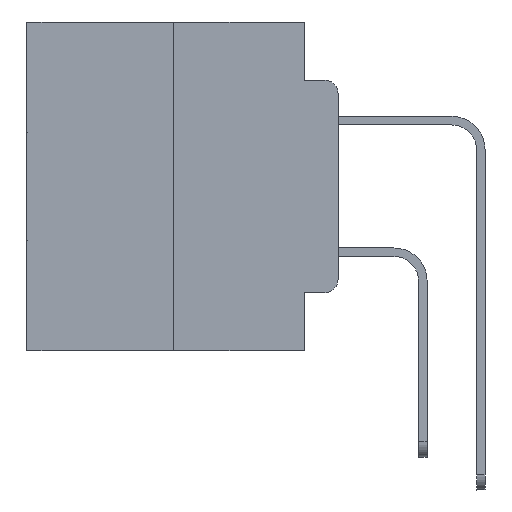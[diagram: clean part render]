
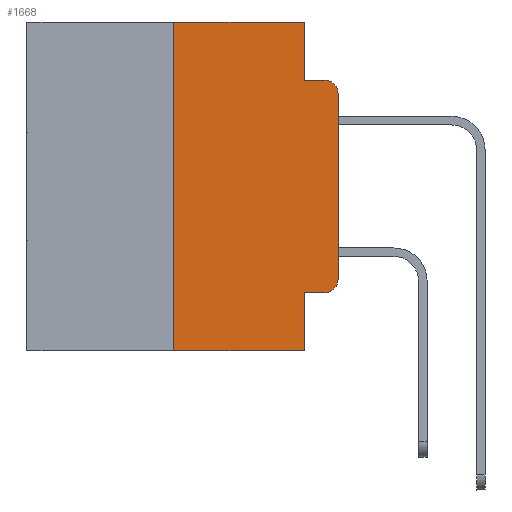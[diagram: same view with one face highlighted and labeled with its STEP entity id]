
A CAD part, left-side view. The second image highlights one B-rep face of the part: STEP entity #1668.
In plain terms, the highlighted planar face has unit normal (-1, 0, 0).
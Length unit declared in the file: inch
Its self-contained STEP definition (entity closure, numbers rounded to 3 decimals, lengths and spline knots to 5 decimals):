
#173 = EDGE_CURVE ( 'NONE', #24649, #8950, #5155, .T. ) ;
#1180 = EDGE_CURVE ( 'NONE', #9304, #15978, #28463, .T. ) ;
#1533 = DIRECTION ( 'NONE',  ( -1., 0., 0. ) ) ;
#1668 = ADVANCED_FACE ( 'NONE', ( #22957 ), #18216, .F. ) ;
#1962 = LINE ( 'NONE', #13817, #7445 ) ;
#1972 = VERTEX_POINT ( 'NONE', #8780 ) ;
#2935 = VERTEX_POINT ( 'NONE', #15382 ) ;
#3604 = CARTESIAN_POINT ( 'NONE',  ( 0., 0.473, -0.5 ) ) ;
#3699 = ORIENTED_EDGE ( 'NONE', *, *, #23379, .T. ) ;
#4369 = LINE ( 'NONE', #8850, #13056 ) ;
#4743 = CARTESIAN_POINT ( 'NONE',  ( 0., 0.051, -0.4115 ) ) ;
#5114 = EDGE_CURVE ( 'NONE', #25478, #2935, #4369, .T. ) ;
#5155 = LINE ( 'NONE', #23146, #24422 ) ;
#5799 = ORIENTED_EDGE ( 'NONE', *, *, #20134, .T. ) ;
#6157 = CIRCLE ( 'NONE', #27824, 0.02 ) ;
#6471 = ORIENTED_EDGE ( 'NONE', *, *, #5114, .F. ) ;
#7056 = LINE ( 'NONE', #4743, #11987 ) ;
#7445 = VECTOR ( 'NONE', #11353, 39.37008 ) ;
#8566 = CARTESIAN_POINT ( 'NONE',  ( 0., 0., -0.3915 ) ) ;
#8761 = CARTESIAN_POINT ( 'NONE',  ( 0., 0.25, -0.5 ) ) ;
#8780 = CARTESIAN_POINT ( 'NONE',  ( 0., 0.051, -0.0885 ) ) ;
#8850 = CARTESIAN_POINT ( 'NONE',  ( 0., 0.25, 0. ) ) ;
#8950 = VERTEX_POINT ( 'NONE', #9825 ) ;
#9304 = VERTEX_POINT ( 'NONE', #21290 ) ;
#9665 = VERTEX_POINT ( 'NONE', #29909 ) ;
#9825 = CARTESIAN_POINT ( 'NONE',  ( 0., 0., -0.1085 ) ) ;
#9832 = ORIENTED_EDGE ( 'NONE', *, *, #17323, .F. ) ;
#10935 = DIRECTION ( 'NONE',  ( 0., 0., -1. ) ) ;
#11316 = DIRECTION ( 'NONE',  ( 0., 0., 1. ) ) ;
#11353 = DIRECTION ( 'NONE',  ( 0., -1., 0. ) ) ;
#11490 = LINE ( 'NONE', #18108, #26871 ) ;
#11987 = VECTOR ( 'NONE', #20879, 39.37008 ) ;
#12619 = CARTESIAN_POINT ( 'NONE',  ( 0., 0.051, 0. ) ) ;
#12716 = ORIENTED_EDGE ( 'NONE', *, *, #1180, .F. ) ;
#13056 = VECTOR ( 'NONE', #11316, 39.37008 ) ;
#13656 = AXIS2_PLACEMENT_3D ( 'NONE', #22585, #1533, #10935 ) ;
#13817 = CARTESIAN_POINT ( 'NONE',  ( 0., 0.051, -0.0885 ) ) ;
#14214 = CARTESIAN_POINT ( 'NONE',  ( 0., 0.051, -0.5 ) ) ;
#14792 = ORIENTED_EDGE ( 'NONE', *, *, #28949, .F. ) ;
#15052 = VERTEX_POINT ( 'NONE', #15418 ) ;
#15382 = CARTESIAN_POINT ( 'NONE',  ( 0., 0.25, 0. ) ) ;
#15418 = CARTESIAN_POINT ( 'NONE',  ( 0., 0.02, -0.0885 ) ) ;
#15453 = DIRECTION ( 'NONE',  ( 1., 0., 0. ) ) ;
#15978 = VERTEX_POINT ( 'NONE', #14214 ) ;
#16047 = CARTESIAN_POINT ( 'NONE',  ( 0., 0.473, 0. ) ) ;
#16765 = CARTESIAN_POINT ( 'NONE',  ( 0., 0.051, 0. ) ) ;
#17323 = EDGE_CURVE ( 'NONE', #1972, #15052, #1962, .T. ) ;
#18108 = CARTESIAN_POINT ( 'NONE',  ( 0., 0.473, 0. ) ) ;
#18216 = PLANE ( 'NONE',  #21245 ) ;
#18865 = ORIENTED_EDGE ( 'NONE', *, *, #23829, .T. ) ;
#18969 = VECTOR ( 'NONE', #27650, 39.37008 ) ;
#19217 = DIRECTION ( 'NONE',  ( 0., 0., -1. ) ) ;
#20134 = EDGE_CURVE ( 'NONE', #9304, #9665, #7056, .T. ) ;
#20541 = LINE ( 'NONE', #29949, #18969 ) ;
#20847 = DIRECTION ( 'NONE',  ( 0., -1., 0. ) ) ;
#20879 = DIRECTION ( 'NONE',  ( 0., -1., 0. ) ) ;
#21245 = AXIS2_PLACEMENT_3D ( 'NONE', #16047, #15453, #27298 ) ;
#21290 = CARTESIAN_POINT ( 'NONE',  ( 0., 0.051, -0.4115 ) ) ;
#21468 = ORIENTED_EDGE ( 'NONE', *, *, #29817, .T. ) ;
#22585 = CARTESIAN_POINT ( 'NONE',  ( 0., 0.02, -0.1085 ) ) ;
#22769 = DIRECTION ( 'NONE',  ( -1., 0., 0. ) ) ;
#22957 = FACE_OUTER_BOUND ( 'NONE', #30298, .T. ) ;
#23146 = CARTESIAN_POINT ( 'NONE',  ( 0., 0., 0. ) ) ;
#23379 = EDGE_CURVE ( 'NONE', #25478, #15978, #26073, .T. ) ;
#23829 = EDGE_CURVE ( 'NONE', #9665, #24649, #6157, .T. ) ;
#23836 = VECTOR ( 'NONE', #28988, 39.37008 ) ;
#24422 = VECTOR ( 'NONE', #30383, 39.37008 ) ;
#24649 = VERTEX_POINT ( 'NONE', #8566 ) ;
#24730 = EDGE_CURVE ( 'NONE', #25354, #1972, #20541, .T. ) ;
#24940 = CARTESIAN_POINT ( 'NONE',  ( 0., 0.02, -0.3915 ) ) ;
#25253 = DIRECTION ( 'NONE',  ( 0., 0., -1. ) ) ;
#25354 = VERTEX_POINT ( 'NONE', #12619 ) ;
#25478 = VERTEX_POINT ( 'NONE', #8761 ) ;
#25914 = ORIENTED_EDGE ( 'NONE', *, *, #173, .T. ) ;
#26073 = LINE ( 'NONE', #3604, #23836 ) ;
#26871 = VECTOR ( 'NONE', #20847, 39.37008 ) ;
#26908 = CIRCLE ( 'NONE', #13656, 0.02 ) ;
#27298 = DIRECTION ( 'NONE',  ( 0., 0., -1. ) ) ;
#27650 = DIRECTION ( 'NONE',  ( 0., 0., -1. ) ) ;
#27824 = AXIS2_PLACEMENT_3D ( 'NONE', #24940, #22769, #25253 ) ;
#28463 = LINE ( 'NONE', #16765, #28611 ) ;
#28611 = VECTOR ( 'NONE', #19217, 39.37008 ) ;
#28814 = ORIENTED_EDGE ( 'NONE', *, *, #24730, .F. ) ;
#28949 = EDGE_CURVE ( 'NONE', #2935, #25354, #11490, .T. ) ;
#28988 = DIRECTION ( 'NONE',  ( 0., -1., 0. ) ) ;
#29817 = EDGE_CURVE ( 'NONE', #8950, #15052, #26908, .T. ) ;
#29909 = CARTESIAN_POINT ( 'NONE',  ( 0., 0.02, -0.4115 ) ) ;
#29949 = CARTESIAN_POINT ( 'NONE',  ( 0., 0.051, 0. ) ) ;
#30298 = EDGE_LOOP ( 'NONE', ( #25914, #21468, #9832, #28814, #14792, #6471, #3699, #12716, #5799, #18865 ) ) ;
#30383 = DIRECTION ( 'NONE',  ( 0., 0., 1. ) ) ;
